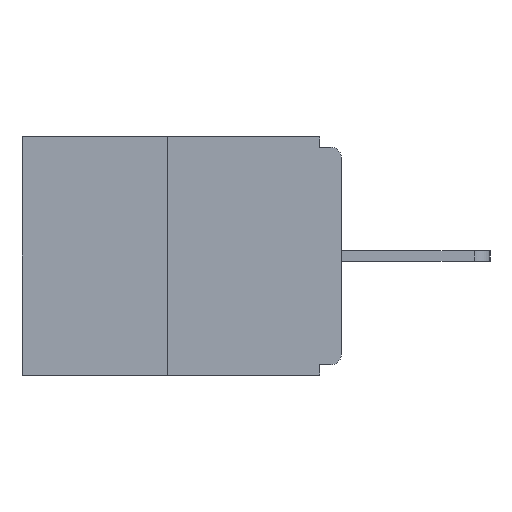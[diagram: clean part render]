
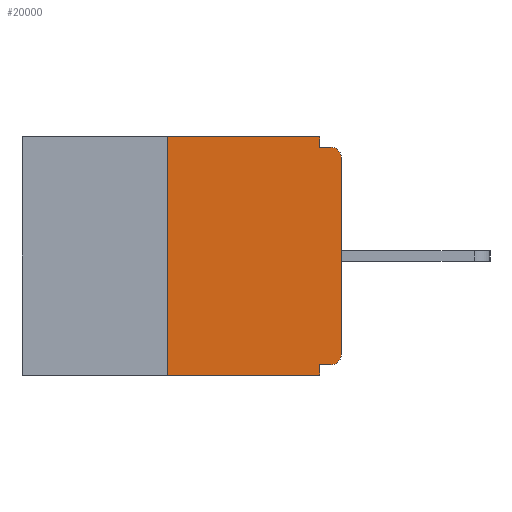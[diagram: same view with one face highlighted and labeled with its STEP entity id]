
A CAD part, left-side view. The second image highlights one B-rep face of the part: STEP entity #20000.
In plain terms, the highlighted planar face has unit normal (-1, 0, 0).
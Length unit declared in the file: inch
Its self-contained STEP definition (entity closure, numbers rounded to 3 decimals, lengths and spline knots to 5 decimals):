
#88 = VERTEX_POINT ( 'NONE', #20961 ) ;
#196 = EDGE_LOOP ( 'NONE', ( #3333, #20321, #2211, #8810, #13524, #2359, #17090, #2346, #20471, #15855 ) ) ;
#216 = VECTOR ( 'NONE', #25486, 39.37008 ) ;
#668 = DIRECTION ( 'NONE',  ( -1., 0., 0. ) ) ;
#1067 = DIRECTION ( 'NONE',  ( 0., 0., 1. ) ) ;
#1157 = EDGE_CURVE ( 'NONE', #2884, #5813, #8594, .T. ) ;
#1846 = DIRECTION ( 'NONE',  ( 0., -1., 0. ) ) ;
#2211 = ORIENTED_EDGE ( 'NONE', *, *, #2916, .T. ) ;
#2330 = CARTESIAN_POINT ( 'NONE',  ( 0., 0.015, -0.328 ) ) ;
#2346 = ORIENTED_EDGE ( 'NONE', *, *, #6570, .T. ) ;
#2359 = ORIENTED_EDGE ( 'NONE', *, *, #6681, .T. ) ;
#2884 = VERTEX_POINT ( 'NONE', #13056 ) ;
#2916 = EDGE_CURVE ( 'NONE', #9385, #5813, #25811, .T. ) ;
#3224 = EDGE_CURVE ( 'NONE', #9385, #17455, #18091, .T. ) ;
#3333 = ORIENTED_EDGE ( 'NONE', *, *, #25368, .F. ) ;
#3549 = CARTESIAN_POINT ( 'NONE',  ( 0., 0.031, -0.343 ) ) ;
#4067 = VECTOR ( 'NONE', #1067, 39.37008 ) ;
#4248 = CARTESIAN_POINT ( 'NONE',  ( 0., 0.25, 0. ) ) ;
#5094 = VERTEX_POINT ( 'NONE', #8000 ) ;
#5345 = DIRECTION ( 'NONE',  ( 0., 0., -1. ) ) ;
#5813 = VERTEX_POINT ( 'NONE', #8733 ) ;
#6395 = VERTEX_POINT ( 'NONE', #24315 ) ;
#6496 = CARTESIAN_POINT ( 'NONE',  ( 0., 0.015, -0.03 ) ) ;
#6570 = EDGE_CURVE ( 'NONE', #88, #6395, #15963, .T. ) ;
#6681 = EDGE_CURVE ( 'NONE', #7740, #5094, #24958, .T. ) ;
#6788 = DIRECTION ( 'NONE',  ( 0., -1., 0. ) ) ;
#7017 = CARTESIAN_POINT ( 'NONE',  ( 0., 0.031, -0.015 ) ) ;
#7104 = DIRECTION ( 'NONE',  ( 0., 0., 1. ) ) ;
#7434 = CARTESIAN_POINT ( 'NONE',  ( 0., 0.031, 0. ) ) ;
#7740 = VERTEX_POINT ( 'NONE', #2330 ) ;
#8000 = CARTESIAN_POINT ( 'NONE',  ( 0., 0., -0.313 ) ) ;
#8579 = DIRECTION ( 'NONE',  ( 0., 0., -1. ) ) ;
#8594 = LINE ( 'NONE', #3549, #23619 ) ;
#8733 = CARTESIAN_POINT ( 'NONE',  ( 0., 0.031, -0.343 ) ) ;
#8810 = ORIENTED_EDGE ( 'NONE', *, *, #1157, .F. ) ;
#8964 = VERTEX_POINT ( 'NONE', #23022 ) ;
#9123 = DIRECTION ( 'NONE',  ( 0., 0., -1. ) ) ;
#9385 = VERTEX_POINT ( 'NONE', #20631 ) ;
#9486 = VECTOR ( 'NONE', #6788, 39.37008 ) ;
#9522 = LINE ( 'NONE', #18317, #14939 ) ;
#9909 = PLANE ( 'NONE',  #18299 ) ;
#11916 = CARTESIAN_POINT ( 'NONE',  ( 0., 0.46, -0.343 ) ) ;
#11975 = DIRECTION ( 'NONE',  ( 1., 0., 0. ) ) ;
#12035 = VECTOR ( 'NONE', #7104, 39.37008 ) ;
#13050 = CARTESIAN_POINT ( 'NONE',  ( 0., 0.015, -0.313 ) ) ;
#13056 = CARTESIAN_POINT ( 'NONE',  ( 0., 0.031, -0.328 ) ) ;
#13112 = AXIS2_PLACEMENT_3D ( 'NONE', #6496, #20781, #8579 ) ;
#13434 = EDGE_CURVE ( 'NONE', #14430, #6395, #16425, .T. ) ;
#13524 = ORIENTED_EDGE ( 'NONE', *, *, #23742, .F. ) ;
#14430 = VERTEX_POINT ( 'NONE', #7017 ) ;
#14939 = VECTOR ( 'NONE', #1846, 39.37008 ) ;
#14976 = FACE_OUTER_BOUND ( 'NONE', #196, .T. ) ;
#15071 = DIRECTION ( 'NONE',  ( 0., 0., -1. ) ) ;
#15168 = CARTESIAN_POINT ( 'NONE',  ( 0., 0.25, 0. ) ) ;
#15855 = ORIENTED_EDGE ( 'NONE', *, *, #19296, .F. ) ;
#15963 = CIRCLE ( 'NONE', #13112, 0.015 ) ;
#16425 = LINE ( 'NONE', #22067, #17716 ) ;
#17090 = ORIENTED_EDGE ( 'NONE', *, *, #24496, .T. ) ;
#17278 = VECTOR ( 'NONE', #5345, 39.37008 ) ;
#17455 = VERTEX_POINT ( 'NONE', #4248 ) ;
#17716 = VECTOR ( 'NONE', #26119, 39.37008 ) ;
#18091 = LINE ( 'NONE', #15168, #12035 ) ;
#18299 = AXIS2_PLACEMENT_3D ( 'NONE', #24206, #11975, #26269 ) ;
#18317 = CARTESIAN_POINT ( 'NONE',  ( 0., 0.46, 0. ) ) ;
#19296 = EDGE_CURVE ( 'NONE', #8964, #14430, #22711, .T. ) ;
#20000 = ADVANCED_FACE ( 'NONE', ( #14976 ), #9909, .F. ) ;
#20321 = ORIENTED_EDGE ( 'NONE', *, *, #3224, .F. ) ;
#20471 = ORIENTED_EDGE ( 'NONE', *, *, #13434, .F. ) ;
#20631 = CARTESIAN_POINT ( 'NONE',  ( 0., 0.25, -0.343 ) ) ;
#20781 = DIRECTION ( 'NONE',  ( -1., 0., 0. ) ) ;
#20961 = CARTESIAN_POINT ( 'NONE',  ( 0., 0., -0.03 ) ) ;
#22058 = LINE ( 'NONE', #23415, #216 ) ;
#22067 = CARTESIAN_POINT ( 'NONE',  ( 0., 0., -0.015 ) ) ;
#22711 = LINE ( 'NONE', #7434, #17278 ) ;
#23022 = CARTESIAN_POINT ( 'NONE',  ( 0., 0.031, 0. ) ) ;
#23415 = CARTESIAN_POINT ( 'NONE',  ( 0., 0., -0.328 ) ) ;
#23619 = VECTOR ( 'NONE', #9123, 39.37008 ) ;
#23742 = EDGE_CURVE ( 'NONE', #7740, #2884, #22058, .T. ) ;
#24206 = CARTESIAN_POINT ( 'NONE',  ( 0., 0.46, 0. ) ) ;
#24315 = CARTESIAN_POINT ( 'NONE',  ( 0., 0.015, -0.015 ) ) ;
#24427 = AXIS2_PLACEMENT_3D ( 'NONE', #13050, #668, #15071 ) ;
#24496 = EDGE_CURVE ( 'NONE', #5094, #88, #25260, .T. ) ;
#24958 = CIRCLE ( 'NONE', #24427, 0.015 ) ;
#25260 = LINE ( 'NONE', #25714, #4067 ) ;
#25368 = EDGE_CURVE ( 'NONE', #17455, #8964, #9522, .T. ) ;
#25486 = DIRECTION ( 'NONE',  ( 0., 1., 0. ) ) ;
#25714 = CARTESIAN_POINT ( 'NONE',  ( 0., 0., 0. ) ) ;
#25811 = LINE ( 'NONE', #11916, #9486 ) ;
#26119 = DIRECTION ( 'NONE',  ( 0., -1., 0. ) ) ;
#26269 = DIRECTION ( 'NONE',  ( 0., 0., -1. ) ) ;
